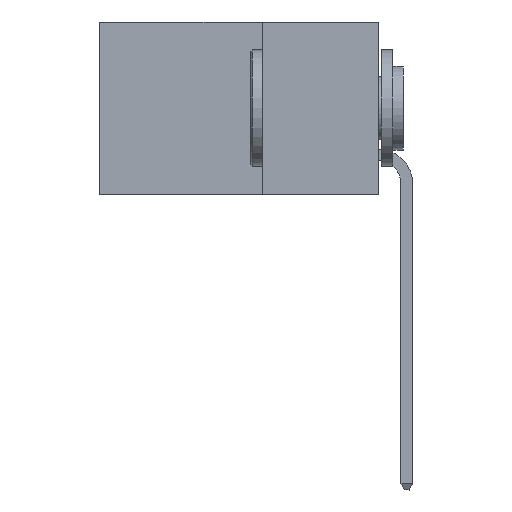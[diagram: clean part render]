
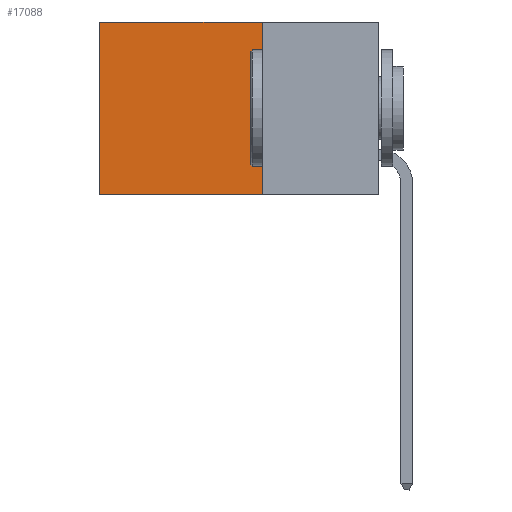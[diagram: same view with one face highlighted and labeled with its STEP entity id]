
A CAD part, left-side view. The second image highlights one B-rep face of the part: STEP entity #17088.
In plain terms, the highlighted planar face has unit normal (-1, 0, 0).
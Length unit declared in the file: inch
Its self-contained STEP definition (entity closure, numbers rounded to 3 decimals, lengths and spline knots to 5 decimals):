
#269 = EDGE_CURVE ( 'NONE', #22949, #11990, #11858, .T. ) ;
#1590 = ORIENTED_EDGE ( 'NONE', *, *, #3362, .F. ) ;
#1919 = DIRECTION ( 'NONE',  ( 1., 0., 0. ) ) ;
#3028 = CARTESIAN_POINT ( 'NONE',  ( 0.298, 0.25, 0. ) ) ;
#3362 = EDGE_CURVE ( 'NONE', #11789, #11990, #17097, .T. ) ;
#3437 = DIRECTION ( 'NONE',  ( 0., 1., 0. ) ) ;
#3624 = CARTESIAN_POINT ( 'NONE',  ( 0.298, 0.6, 0. ) ) ;
#6101 = DIRECTION ( 'NONE',  ( 0., 0., -1. ) ) ;
#8015 = ORIENTED_EDGE ( 'NONE', *, *, #26871, .T. ) ;
#8145 = VECTOR ( 'NONE', #19228, 39.37008 ) ;
#8880 = LINE ( 'NONE', #26177, #8145 ) ;
#10775 = CARTESIAN_POINT ( 'NONE',  ( 0.298, 0.6, 0. ) ) ;
#11182 = PLANE ( 'NONE',  #24955 ) ;
#11265 = VERTEX_POINT ( 'NONE', #3028 ) ;
#11301 = EDGE_LOOP ( 'NONE', ( #26928, #1590, #27866, #8015 ) ) ;
#11326 = CARTESIAN_POINT ( 'NONE',  ( 0.298, 0.25, -0.37 ) ) ;
#11789 = VERTEX_POINT ( 'NONE', #11326 ) ;
#11858 = LINE ( 'NONE', #10775, #13650 ) ;
#11990 = VERTEX_POINT ( 'NONE', #16610 ) ;
#13650 = VECTOR ( 'NONE', #6101, 39.37008 ) ;
#15746 = EDGE_CURVE ( 'NONE', #11265, #11789, #8880, .T. ) ;
#15866 = CARTESIAN_POINT ( 'NONE',  ( 0.298, 0.25, 0. ) ) ;
#16413 = FACE_OUTER_BOUND ( 'NONE', #11301, .T. ) ;
#16610 = CARTESIAN_POINT ( 'NONE',  ( 0.298, 0.6, -0.37 ) ) ;
#17088 = ADVANCED_FACE ( 'NONE', ( #16413 ), #11182, .F. ) ;
#17097 = LINE ( 'NONE', #27023, #19271 ) ;
#19228 = DIRECTION ( 'NONE',  ( 0., 0., -1. ) ) ;
#19271 = VECTOR ( 'NONE', #3437, 39.37008 ) ;
#20010 = DIRECTION ( 'NONE',  ( 0., 0., -1. ) ) ;
#22949 = VERTEX_POINT ( 'NONE', #3624 ) ;
#22979 = CARTESIAN_POINT ( 'NONE',  ( 0.298, 0.25, 0. ) ) ;
#24955 = AXIS2_PLACEMENT_3D ( 'NONE', #15866, #1919, #20010 ) ;
#25030 = DIRECTION ( 'NONE',  ( 0., 1., 0. ) ) ;
#26038 = LINE ( 'NONE', #22979, #27499 ) ;
#26177 = CARTESIAN_POINT ( 'NONE',  ( 0.298, 0.25, 0. ) ) ;
#26871 = EDGE_CURVE ( 'NONE', #11265, #22949, #26038, .T. ) ;
#26928 = ORIENTED_EDGE ( 'NONE', *, *, #269, .T. ) ;
#27023 = CARTESIAN_POINT ( 'NONE',  ( 0.298, 0.25, -0.37 ) ) ;
#27499 = VECTOR ( 'NONE', #25030, 39.37008 ) ;
#27866 = ORIENTED_EDGE ( 'NONE', *, *, #15746, .F. ) ;
